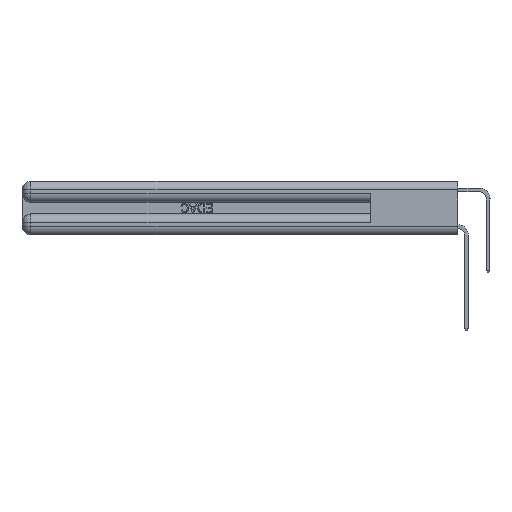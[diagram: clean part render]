
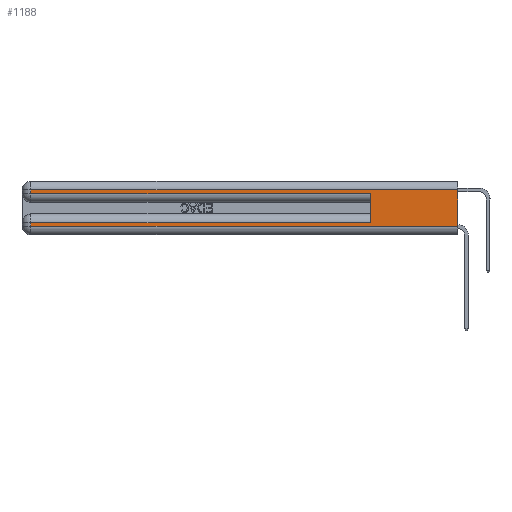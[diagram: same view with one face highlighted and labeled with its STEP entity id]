
A CAD part, left-side view. The second image highlights one B-rep face of the part: STEP entity #1188.
In plain terms, the highlighted planar face has unit normal (-1, 0, 0).
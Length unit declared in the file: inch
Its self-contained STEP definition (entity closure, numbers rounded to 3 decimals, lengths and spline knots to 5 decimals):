
#1188 = ADVANCED_FACE ( 'NONE', ( #9775 ), #34005, .F. ) ;
#1878 = CARTESIAN_POINT ( 'NONE',  ( 0., 2.94, 0.285 ) ) ;
#2325 = AXIS2_PLACEMENT_3D ( 'NONE', #8010, #37044, #25218 ) ;
#3174 = VERTEX_POINT ( 'NONE', #7355 ) ;
#7233 = EDGE_CURVE ( 'NONE', #23725, #32894, #27522, .T. ) ;
#7355 = CARTESIAN_POINT ( 'NONE',  ( 0., 0.6, 0.285 ) ) ;
#7436 = VERTEX_POINT ( 'NONE', #35958 ) ;
#7922 = VERTEX_POINT ( 'NONE', #24269 ) ;
#8010 = CARTESIAN_POINT ( 'NONE',  ( 0., 0., 0.37 ) ) ;
#8055 = VECTOR ( 'NONE', #32294, 39.37008 ) ;
#8278 = ORIENTED_EDGE ( 'NONE', *, *, #24618, .F. ) ;
#8463 = EDGE_CURVE ( 'NONE', #24716, #17326, #24717, .T. ) ;
#8490 = CARTESIAN_POINT ( 'NONE',  ( 0., 0., 0.31 ) ) ;
#8649 = CARTESIAN_POINT ( 'NONE',  ( 0., 2.94, 0.085 ) ) ;
#9600 = CARTESIAN_POINT ( 'NONE',  ( 0., 0., 0.37 ) ) ;
#9775 = FACE_OUTER_BOUND ( 'NONE', #31210, .T. ) ;
#10075 = LINE ( 'NONE', #15283, #31366 ) ;
#11359 = CARTESIAN_POINT ( 'NONE',  ( 0., 0.6, 0.145 ) ) ;
#11493 = EDGE_CURVE ( 'NONE', #32034, #7436, #33128, .T. ) ;
#11642 = LINE ( 'NONE', #15317, #36182 ) ;
#11999 = CARTESIAN_POINT ( 'NONE',  ( 0., 0., 0.085 ) ) ;
#13841 = ORIENTED_EDGE ( 'NONE', *, *, #29432, .T. ) ;
#15283 = CARTESIAN_POINT ( 'NONE',  ( 0., 0., 0.06 ) ) ;
#15317 = CARTESIAN_POINT ( 'NONE',  ( 0., 2.94, 0.37 ) ) ;
#15903 = DIRECTION ( 'NONE',  ( 0., 0., -1. ) ) ;
#17203 = CARTESIAN_POINT ( 'NONE',  ( 0., 0.6, 0.085 ) ) ;
#17326 = VERTEX_POINT ( 'NONE', #1878 ) ;
#17759 = CARTESIAN_POINT ( 'NONE',  ( 0., 2.94, 0.31 ) ) ;
#18099 = DIRECTION ( 'NONE',  ( 0., 0., -1. ) ) ;
#19739 = DIRECTION ( 'NONE',  ( 0., 1., 0. ) ) ;
#20563 = EDGE_CURVE ( 'NONE', #32894, #7922, #11642, .T. ) ;
#21043 = DIRECTION ( 'NONE',  ( 0., -1., 0. ) ) ;
#21069 = ORIENTED_EDGE ( 'NONE', *, *, #7233, .T. ) ;
#21581 = ORIENTED_EDGE ( 'NONE', *, *, #23962, .T. ) ;
#23725 = VERTEX_POINT ( 'NONE', #17203 ) ;
#23921 = ORIENTED_EDGE ( 'NONE', *, *, #8463, .T. ) ;
#23937 = DIRECTION ( 'NONE',  ( 0., -1., 0. ) ) ;
#23962 = EDGE_CURVE ( 'NONE', #7922, #7436, #10075, .T. ) ;
#24269 = CARTESIAN_POINT ( 'NONE',  ( 0., 2.94, 0.06 ) ) ;
#24618 = EDGE_CURVE ( 'NONE', #23725, #3174, #30447, .T. ) ;
#24716 = VERTEX_POINT ( 'NONE', #17759 ) ;
#24717 = LINE ( 'NONE', #36521, #28365 ) ;
#25218 = DIRECTION ( 'NONE',  ( 0., 0., -1. ) ) ;
#27522 = LINE ( 'NONE', #11999, #8055 ) ;
#27823 = VECTOR ( 'NONE', #21043, 39.37008 ) ;
#27900 = ORIENTED_EDGE ( 'NONE', *, *, #11493, .F. ) ;
#27972 = CARTESIAN_POINT ( 'NONE',  ( 0., 0., 0.31 ) ) ;
#28365 = VECTOR ( 'NONE', #33718, 39.37008 ) ;
#29008 = VECTOR ( 'NONE', #15903, 39.37008 ) ;
#29289 = VECTOR ( 'NONE', #19739, 39.37008 ) ;
#29432 = EDGE_CURVE ( 'NONE', #17326, #3174, #35560, .T. ) ;
#30447 = LINE ( 'NONE', #11359, #35493 ) ;
#30914 = ORIENTED_EDGE ( 'NONE', *, *, #33432, .T. ) ;
#31210 = EDGE_LOOP ( 'NONE', ( #27900, #30914, #23921, #13841, #8278, #21069, #32323, #21581 ) ) ;
#31366 = VECTOR ( 'NONE', #23937, 39.37008 ) ;
#32034 = VERTEX_POINT ( 'NONE', #27972 ) ;
#32294 = DIRECTION ( 'NONE',  ( 0., 1., 0. ) ) ;
#32323 = ORIENTED_EDGE ( 'NONE', *, *, #20563, .T. ) ;
#32894 = VERTEX_POINT ( 'NONE', #8649 ) ;
#33128 = LINE ( 'NONE', #9600, #29008 ) ;
#33432 = EDGE_CURVE ( 'NONE', #32034, #24716, #37060, .T. ) ;
#33718 = DIRECTION ( 'NONE',  ( 0., 0., -1. ) ) ;
#34005 = PLANE ( 'NONE',  #2325 ) ;
#34584 = DIRECTION ( 'NONE',  ( 0., 0., 1. ) ) ;
#35493 = VECTOR ( 'NONE', #34584, 39.37008 ) ;
#35549 = CARTESIAN_POINT ( 'NONE',  ( 0., 0., 0.285 ) ) ;
#35560 = LINE ( 'NONE', #35549, #27823 ) ;
#35958 = CARTESIAN_POINT ( 'NONE',  ( 0., 0., 0.06 ) ) ;
#36182 = VECTOR ( 'NONE', #18099, 39.37008 ) ;
#36521 = CARTESIAN_POINT ( 'NONE',  ( 0., 2.94, 0.37 ) ) ;
#37044 = DIRECTION ( 'NONE',  ( 1., 0., 0. ) ) ;
#37060 = LINE ( 'NONE', #8490, #29289 ) ;
